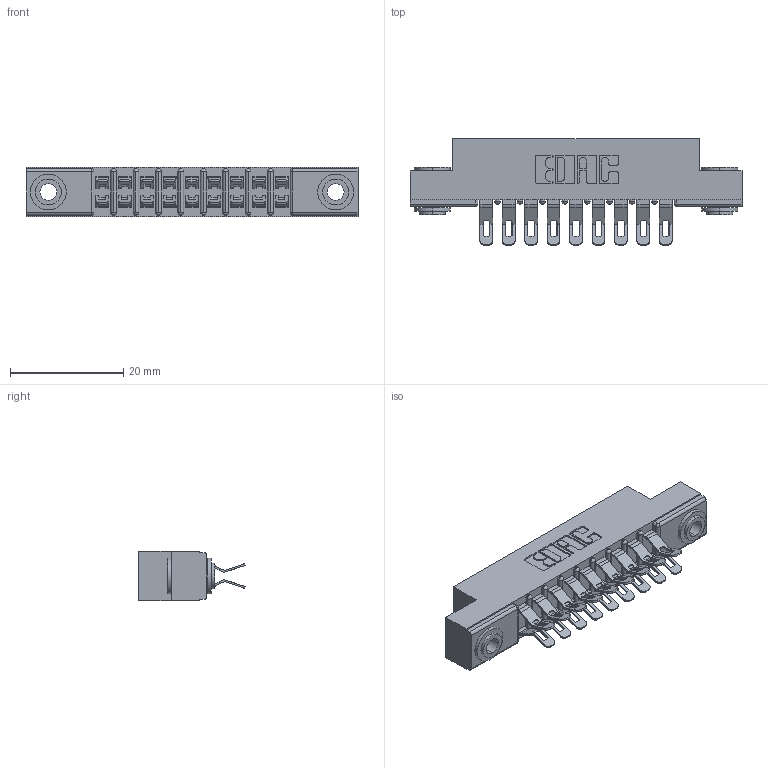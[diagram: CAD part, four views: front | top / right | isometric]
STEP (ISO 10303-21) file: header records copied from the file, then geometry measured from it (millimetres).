
FILE_DESCRIPTION (( 'STEP AP203' ), '1' );
FILE_NAME ('357-018-455-203.STEP', '2020-10-02T20:44:18', ( '' ), ( '' ), 'SwSTEP 2.0', 'SolidWorks 2020', '' );
FILE_SCHEMA (( 'CONFIG_CONTROL_DESIGN' ));
Length unit declared in the file: inch
Products named in the file (4): 307 Part_.156 Dia Mounting Holes; 357-018-455-203; 307-290-001_555; 345-250-002_345-250-002-102
Assembly tree (21 placements, depth 2):
  357-018-455-203
    307 Part_.156 Dia Mounting Holes
    307-290-001_555  x18
    345-250-002_345-250-002-102  x2
Bounding box: 58.67 x 18.75 x 8.71 mm (x, y, z)
Volume: 3894.3 mm3; surface area: 6743.8 mm2
Topology: 21 solids, 21 shells, 1278 faces, 3693 edges, 2406 vertices
Faces by surface type: plane 706, cylinder 544, sphere 20, cone 8
Entity records: 13674 total; most frequent: CARTESIAN_POINT 2234, DIRECTION 2224, ORIENTED_EDGE 2204, EDGE_CURVE 1102, VECTOR 812, LINE 812, VERTEX_POINT 716, AXIS2_PLACEMENT_3D 706
